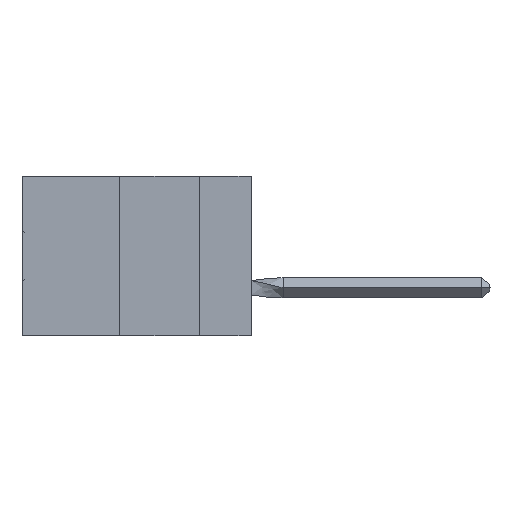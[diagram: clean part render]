
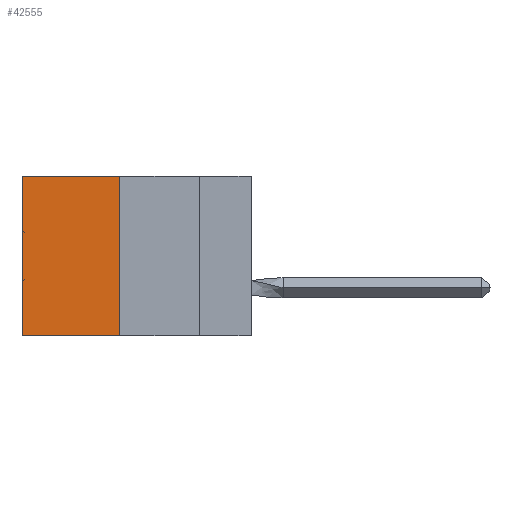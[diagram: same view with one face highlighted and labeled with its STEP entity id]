
A CAD part, left-side view. The second image highlights one B-rep face of the part: STEP entity #42555.
In plain terms, the highlighted planar face has unit normal (-1, 0, 0).
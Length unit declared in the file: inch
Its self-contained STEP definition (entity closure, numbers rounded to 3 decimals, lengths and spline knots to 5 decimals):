
#1087 = CARTESIAN_POINT ( 'NONE',  ( 0.305, 0.72, -0.5 ) ) ;
#5054 = ORIENTED_EDGE ( 'NONE', *, *, #39619, .T. ) ;
#5940 = CARTESIAN_POINT ( 'NONE',  ( 0.305, 0.72, -0.5 ) ) ;
#6994 = EDGE_CURVE ( 'NONE', #29916, #17550, #14277, .T. ) ;
#7688 = VECTOR ( 'NONE', #49795, 39.37008 ) ;
#7902 = DIRECTION ( 'NONE',  ( 0., 0., -1. ) ) ;
#8826 = CARTESIAN_POINT ( 'NONE',  ( 0.305, 0.413, 0. ) ) ;
#11877 = ORIENTED_EDGE ( 'NONE', *, *, #6994, .F. ) ;
#14277 = LINE ( 'NONE', #24394, #33526 ) ;
#15565 = CARTESIAN_POINT ( 'NONE',  ( 0.305, 0.413, -0.5 ) ) ;
#15732 = ORIENTED_EDGE ( 'NONE', *, *, #29848, .F. ) ;
#15968 = LINE ( 'NONE', #5940, #35111 ) ;
#17550 = VERTEX_POINT ( 'NONE', #1087 ) ;
#18873 = VECTOR ( 'NONE', #31542, 39.37008 ) ;
#20089 = CARTESIAN_POINT ( 'NONE',  ( 0.305, 0.413, -0.5 ) ) ;
#22985 = EDGE_CURVE ( 'NONE', #23255, #26478, #25059, .T. ) ;
#23255 = VERTEX_POINT ( 'NONE', #52755 ) ;
#24295 = ORIENTED_EDGE ( 'NONE', *, *, #22985, .T. ) ;
#24394 = CARTESIAN_POINT ( 'NONE',  ( 0.305, 0.413, -0.5 ) ) ;
#25059 = LINE ( 'NONE', #8826, #7688 ) ;
#26478 = VERTEX_POINT ( 'NONE', #47244 ) ;
#29821 = LINE ( 'NONE', #48047, #18873 ) ;
#29848 = EDGE_CURVE ( 'NONE', #23255, #29916, #29821, .T. ) ;
#29916 = VERTEX_POINT ( 'NONE', #15565 ) ;
#30476 = AXIS2_PLACEMENT_3D ( 'NONE', #20089, #52814, #7902 ) ;
#31542 = DIRECTION ( 'NONE',  ( 0., 0., -1. ) ) ;
#33526 = VECTOR ( 'NONE', #53139, 39.37008 ) ;
#34596 = DIRECTION ( 'NONE',  ( 0., 0., -1. ) ) ;
#35111 = VECTOR ( 'NONE', #34596, 39.37008 ) ;
#36187 = PLANE ( 'NONE',  #30476 ) ;
#39619 = EDGE_CURVE ( 'NONE', #26478, #17550, #15968, .T. ) ;
#42555 = ADVANCED_FACE ( 'NONE', ( #44479 ), #36187, .F. ) ;
#44479 = FACE_OUTER_BOUND ( 'NONE', #50141, .T. ) ;
#47244 = CARTESIAN_POINT ( 'NONE',  ( 0.305, 0.72, 0. ) ) ;
#48047 = CARTESIAN_POINT ( 'NONE',  ( 0.305, 0.413, -0.5 ) ) ;
#49795 = DIRECTION ( 'NONE',  ( 0., 1., 0. ) ) ;
#50141 = EDGE_LOOP ( 'NONE', ( #5054, #11877, #15732, #24295 ) ) ;
#52755 = CARTESIAN_POINT ( 'NONE',  ( 0.305, 0.413, 0. ) ) ;
#52814 = DIRECTION ( 'NONE',  ( 1., 0., 0. ) ) ;
#53139 = DIRECTION ( 'NONE',  ( 0., 1., 0. ) ) ;
